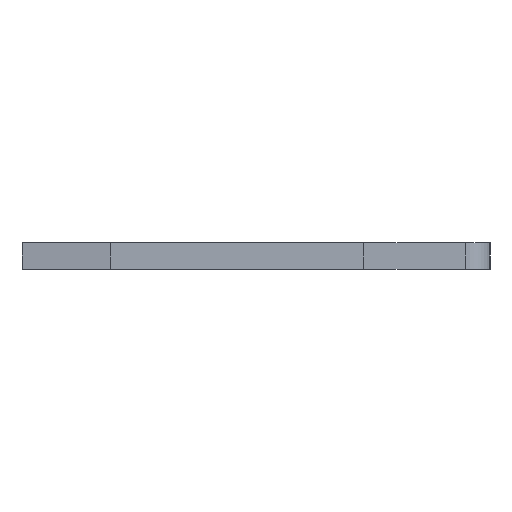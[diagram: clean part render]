
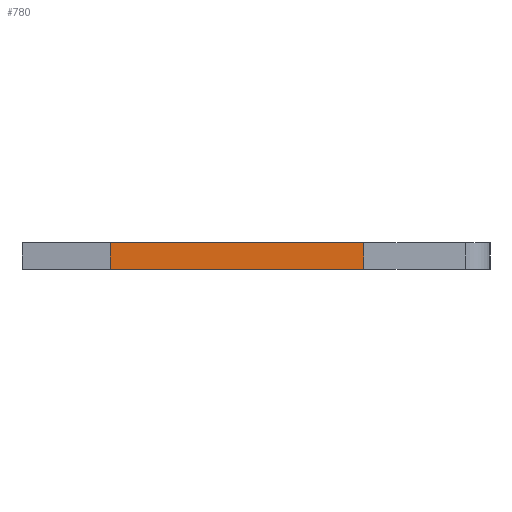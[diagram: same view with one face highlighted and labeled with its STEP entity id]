
A CAD part, left-side view. The second image highlights one B-rep face of the part: STEP entity #780.
In plain terms, the highlighted face is planar.
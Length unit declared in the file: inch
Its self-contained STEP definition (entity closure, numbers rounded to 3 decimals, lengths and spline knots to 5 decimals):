
#2 = EDGE_CURVE ( 'NONE', #1057, #1025, #894, .T. ) ;
#16 = VECTOR ( 'NONE', #995, 39.37008 ) ;
#68 = EDGE_CURVE ( 'NONE', #782, #1025, #853, .T. ) ;
#72 = CARTESIAN_POINT ( 'NONE',  ( -0.013, 0.146, -0.0575 ) ) ;
#81 = PLANE ( 'NONE',  #919 ) ;
#82 = ORIENTED_EDGE ( 'NONE', *, *, #630, .T. ) ;
#133 = VECTOR ( 'NONE', #496, 39.37008 ) ;
#177 = ORIENTED_EDGE ( 'NONE', *, *, #459, .F. ) ;
#274 = LINE ( 'NONE', #978, #133 ) ;
#288 = LINE ( 'NONE', #337, #16 ) ;
#337 = CARTESIAN_POINT ( 'NONE',  ( 0.013, -0.099, -0.0575 ) ) ;
#445 = ORIENTED_EDGE ( 'NONE', *, *, #68, .F. ) ;
#447 = DIRECTION ( 'NONE',  ( 0., 1., 0. ) ) ;
#452 = DIRECTION ( 'NONE',  ( 1., 0., 0. ) ) ;
#459 = EDGE_CURVE ( 'NONE', #761, #782, #274, .T. ) ;
#496 = DIRECTION ( 'NONE',  ( 0., 1., 0. ) ) ;
#538 = ORIENTED_EDGE ( 'NONE', *, *, #2, .T. ) ;
#548 = CARTESIAN_POINT ( 'NONE',  ( -0.013, 0.146, -0.0575 ) ) ;
#561 = VECTOR ( 'NONE', #447, 39.37008 ) ;
#629 = CARTESIAN_POINT ( 'NONE',  ( 0.013, -0.099, -0.0575 ) ) ;
#630 = EDGE_CURVE ( 'NONE', #761, #1057, #288, .T. ) ;
#740 = DIRECTION ( 'NONE',  ( -1., 0., 0. ) ) ;
#753 = EDGE_LOOP ( 'NONE', ( #538, #445, #177, #82 ) ) ;
#761 = VERTEX_POINT ( 'NONE', #629 ) ;
#780 = ADVANCED_FACE ( 'NONE', ( #960 ), #81, .F. ) ;
#782 = VERTEX_POINT ( 'NONE', #1012 ) ;
#822 = VECTOR ( 'NONE', #740, 39.37008 ) ;
#823 = CARTESIAN_POINT ( 'NONE',  ( 0.013, 0.146, -0.0575 ) ) ;
#828 = DIRECTION ( 'NONE',  ( 0., 0., 1. ) ) ;
#853 = LINE ( 'NONE', #823, #822 ) ;
#894 = LINE ( 'NONE', #72, #561 ) ;
#919 = AXIS2_PLACEMENT_3D ( 'NONE', #1213, #828, #452 ) ;
#960 = FACE_OUTER_BOUND ( 'NONE', #753, .T. ) ;
#978 = CARTESIAN_POINT ( 'NONE',  ( 0.013, 0.146, -0.0575 ) ) ;
#995 = DIRECTION ( 'NONE',  ( -1., 0., 0. ) ) ;
#1012 = CARTESIAN_POINT ( 'NONE',  ( 0.013, 0.146, -0.0575 ) ) ;
#1025 = VERTEX_POINT ( 'NONE', #548 ) ;
#1040 = CARTESIAN_POINT ( 'NONE',  ( -0.013, -0.099, -0.0575 ) ) ;
#1057 = VERTEX_POINT ( 'NONE', #1040 ) ;
#1213 = CARTESIAN_POINT ( 'NONE',  ( 0.013, 0.146, -0.0575 ) ) ;
